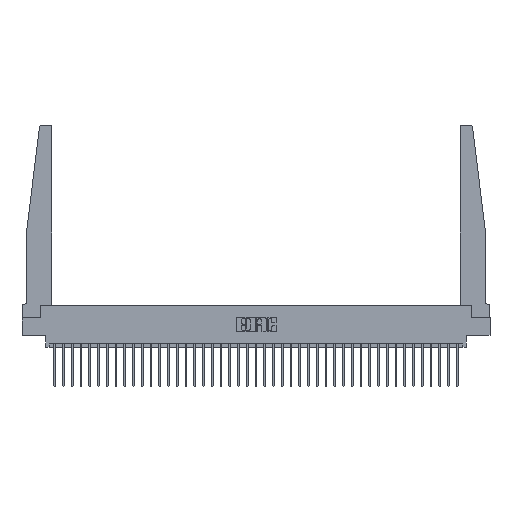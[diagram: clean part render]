
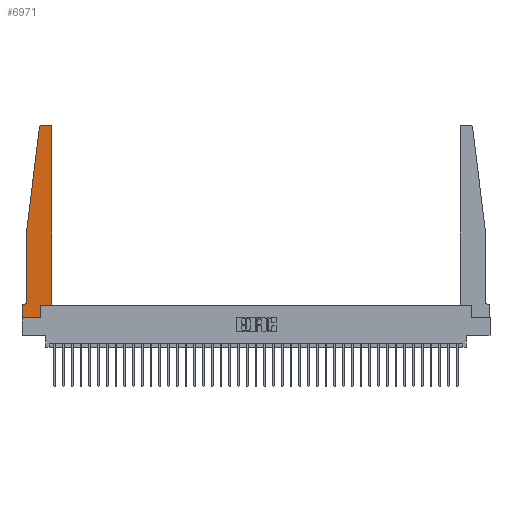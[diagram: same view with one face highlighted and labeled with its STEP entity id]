
A CAD part, top view. The second image highlights one B-rep face of the part: STEP entity #6971.
In plain terms, the highlighted planar face has unit normal (0, 0, 1).
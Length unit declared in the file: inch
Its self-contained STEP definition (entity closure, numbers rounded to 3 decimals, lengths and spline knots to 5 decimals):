
#205 = VERTEX_POINT ( 'NONE', #6828 ) ;
#639 = CARTESIAN_POINT ( 'NONE',  ( 0.395, 2.75, 0.37 ) ) ;
#892 = DIRECTION ( 'NONE',  ( 0., 0., -1. ) ) ;
#947 = DIRECTION ( 'NONE',  ( 0., 0., 1. ) ) ;
#1250 = LINE ( 'NONE', #12218, #21254 ) ;
#1431 = DIRECTION ( 'NONE',  ( -1., 0., 0. ) ) ;
#1709 = EDGE_CURVE ( 'NONE', #28012, #18119, #16448, .T. ) ;
#2001 = ORIENTED_EDGE ( 'NONE', *, *, #11973, .T. ) ;
#2276 = LINE ( 'NONE', #28451, #8669 ) ;
#2583 = EDGE_CURVE ( 'NONE', #34535, #3404, #32292, .T. ) ;
#3404 = VERTEX_POINT ( 'NONE', #10904 ) ;
#4847 = LINE ( 'NONE', #20778, #24781 ) ;
#4904 = DIRECTION ( 'NONE',  ( 0., -1., 0. ) ) ;
#5027 = AXIS2_PLACEMENT_3D ( 'NONE', #17305, #947, #20009 ) ;
#5365 = EDGE_CURVE ( 'NONE', #18119, #19310, #1250, .T. ) ;
#6057 = EDGE_CURVE ( 'NONE', #6517, #34535, #23319, .T. ) ;
#6517 = VERTEX_POINT ( 'NONE', #7039 ) ;
#6828 = CARTESIAN_POINT ( 'NONE',  ( 0.27653, 2.75, 0.37 ) ) ;
#6971 = ADVANCED_FACE ( 'NONE', ( #18242 ), #22433, .T. ) ;
#7039 = CARTESIAN_POINT ( 'NONE',  ( 0., 0.1875, 0.37 ) ) ;
#7357 = DIRECTION ( 'NONE',  ( 0., -1., 0. ) ) ;
#7361 = VECTOR ( 'NONE', #8537, 39.37008 ) ;
#7578 = ORIENTED_EDGE ( 'NONE', *, *, #15210, .T. ) ;
#7621 = VERTEX_POINT ( 'NONE', #639 ) ;
#8324 = VECTOR ( 'NONE', #18068, 39.37008 ) ;
#8334 = EDGE_CURVE ( 'NONE', #205, #20169, #28629, .T. ) ;
#8537 = DIRECTION ( 'NONE',  ( 0., 1., 0. ) ) ;
#8669 = VECTOR ( 'NONE', #1431, 39.37008 ) ;
#8680 = DIRECTION ( 'NONE',  ( -0.122, -0.992, 0. ) ) ;
#8867 = VECTOR ( 'NONE', #4904, 39.37008 ) ;
#9219 = EDGE_CURVE ( 'NONE', #7621, #205, #2276, .T. ) ;
#9268 = CARTESIAN_POINT ( 'NONE',  ( 0.395, 2.72, 0.37 ) ) ;
#9692 = ORIENTED_EDGE ( 'NONE', *, *, #30905, .T. ) ;
#10163 = EDGE_CURVE ( 'NONE', #32130, #15969, #17604, .T. ) ;
#10904 = CARTESIAN_POINT ( 'NONE',  ( 0.2605, 0., 0.37 ) ) ;
#11620 = DIRECTION ( 'NONE',  ( 0., 0., 1. ) ) ;
#11873 = CARTESIAN_POINT ( 'NONE',  ( 0.24675, 2.72367, 0.37 ) ) ;
#11973 = EDGE_CURVE ( 'NONE', #19310, #7621, #18926, .T. ) ;
#11998 = DIRECTION ( 'NONE',  ( 1., 0., 0. ) ) ;
#12218 = CARTESIAN_POINT ( 'NONE',  ( 0.425, 0.18, 0.37 ) ) ;
#13719 = LINE ( 'NONE', #24764, #7361 ) ;
#14112 = CARTESIAN_POINT ( 'NONE',  ( 0.015, 0.1875, 0.37 ) ) ;
#15200 = AXIS2_PLACEMENT_3D ( 'NONE', #9268, #28174, #11998 ) ;
#15210 = EDGE_CURVE ( 'NONE', #3404, #28012, #13719, .T. ) ;
#15321 = CARTESIAN_POINT ( 'NONE',  ( 0.425, 0.18, 0.37 ) ) ;
#15687 = ORIENTED_EDGE ( 'NONE', *, *, #1709, .T. ) ;
#15844 = CARTESIAN_POINT ( 'NONE',  ( 0.065, 0.1875, 0.37 ) ) ;
#15969 = VERTEX_POINT ( 'NONE', #14112 ) ;
#16090 = ORIENTED_EDGE ( 'NONE', *, *, #9219, .T. ) ;
#16289 = CARTESIAN_POINT ( 'NONE',  ( 0., 0., 0.37 ) ) ;
#16448 = LINE ( 'NONE', #15321, #8324 ) ;
#16895 = AXIS2_PLACEMENT_3D ( 'NONE', #27795, #11620, #30466 ) ;
#16898 = EDGE_LOOP ( 'NONE', ( #16090, #23260, #9692, #32019, #26603, #33683, #21173, #28277, #7578, #15687, #22855, #2001 ) ) ;
#17189 = CARTESIAN_POINT ( 'NONE',  ( 0.2605, 0.18, 0.37 ) ) ;
#17251 = CARTESIAN_POINT ( 'NONE',  ( 0.015, 0.2375, 0.37 ) ) ;
#17305 = CARTESIAN_POINT ( 'NONE',  ( 0.27653, 2.72, 0.37 ) ) ;
#17604 = CIRCLE ( 'NONE', #19887, 0.05 ) ;
#17778 = CARTESIAN_POINT ( 'NONE',  ( 0.065, 1.25, 0.37 ) ) ;
#18068 = DIRECTION ( 'NONE',  ( 1., 0., 0. ) ) ;
#18119 = VERTEX_POINT ( 'NONE', #29802 ) ;
#18242 = FACE_OUTER_BOUND ( 'NONE', #16898, .T. ) ;
#18839 = LINE ( 'NONE', #30967, #33038 ) ;
#18926 = CIRCLE ( 'NONE', #15200, 0.03 ) ;
#19310 = VERTEX_POINT ( 'NONE', #34702 ) ;
#19887 = AXIS2_PLACEMENT_3D ( 'NONE', #17251, #892, #19949 ) ;
#19949 = DIRECTION ( 'NONE',  ( -1., 0., 0. ) ) ;
#20009 = DIRECTION ( 'NONE',  ( 1., 0., 0. ) ) ;
#20169 = VERTEX_POINT ( 'NONE', #11873 ) ;
#20778 = CARTESIAN_POINT ( 'NONE',  ( 0.065, 1.25, 0.37 ) ) ;
#21173 = ORIENTED_EDGE ( 'NONE', *, *, #6057, .T. ) ;
#21254 = VECTOR ( 'NONE', #33736, 39.37008 ) ;
#21472 = LINE ( 'NONE', #15844, #24000 ) ;
#22433 = PLANE ( 'NONE',  #16895 ) ;
#22609 = CARTESIAN_POINT ( 'NONE',  ( 0., 0., 0.37 ) ) ;
#22855 = ORIENTED_EDGE ( 'NONE', *, *, #5365, .T. ) ;
#23260 = ORIENTED_EDGE ( 'NONE', *, *, #8334, .T. ) ;
#23319 = LINE ( 'NONE', #23894, #8867 ) ;
#23559 = EDGE_CURVE ( 'NONE', #15969, #6517, #21472, .T. ) ;
#23894 = CARTESIAN_POINT ( 'NONE',  ( 0., 0., 0.37 ) ) ;
#24000 = VECTOR ( 'NONE', #31882, 39.37008 ) ;
#24377 = VECTOR ( 'NONE', #30634, 39.37008 ) ;
#24764 = CARTESIAN_POINT ( 'NONE',  ( 0.2605, 0.18, 0.37 ) ) ;
#24781 = VECTOR ( 'NONE', #7357, 39.37008 ) ;
#26603 = ORIENTED_EDGE ( 'NONE', *, *, #10163, .T. ) ;
#27795 = CARTESIAN_POINT ( 'NONE',  ( 0., 0.1875, 0.37 ) ) ;
#28012 = VERTEX_POINT ( 'NONE', #17189 ) ;
#28174 = DIRECTION ( 'NONE',  ( 0., 0., 1. ) ) ;
#28277 = ORIENTED_EDGE ( 'NONE', *, *, #2583, .T. ) ;
#28451 = CARTESIAN_POINT ( 'NONE',  ( 0.25, 2.75, 0.37 ) ) ;
#28629 = CIRCLE ( 'NONE', #5027, 0.03 ) ;
#29795 = EDGE_CURVE ( 'NONE', #30961, #32130, #4847, .T. ) ;
#29802 = CARTESIAN_POINT ( 'NONE',  ( 0.425, 0.18, 0.37 ) ) ;
#30466 = DIRECTION ( 'NONE',  ( 1., 0., 0. ) ) ;
#30634 = DIRECTION ( 'NONE',  ( 1., 0., 0. ) ) ;
#30905 = EDGE_CURVE ( 'NONE', #20169, #30961, #18839, .T. ) ;
#30961 = VERTEX_POINT ( 'NONE', #17778 ) ;
#30967 = CARTESIAN_POINT ( 'NONE',  ( 0.065, 1.25, 0.37 ) ) ;
#31882 = DIRECTION ( 'NONE',  ( -1., 0., 0. ) ) ;
#32019 = ORIENTED_EDGE ( 'NONE', *, *, #29795, .T. ) ;
#32130 = VERTEX_POINT ( 'NONE', #32930 ) ;
#32292 = LINE ( 'NONE', #22609, #24377 ) ;
#32930 = CARTESIAN_POINT ( 'NONE',  ( 0.065, 0.2375, 0.37 ) ) ;
#33038 = VECTOR ( 'NONE', #8680, 39.37008 ) ;
#33683 = ORIENTED_EDGE ( 'NONE', *, *, #23559, .T. ) ;
#33736 = DIRECTION ( 'NONE',  ( 0., 1., 0. ) ) ;
#34535 = VERTEX_POINT ( 'NONE', #16289 ) ;
#34702 = CARTESIAN_POINT ( 'NONE',  ( 0.425, 2.72, 0.37 ) ) ;
